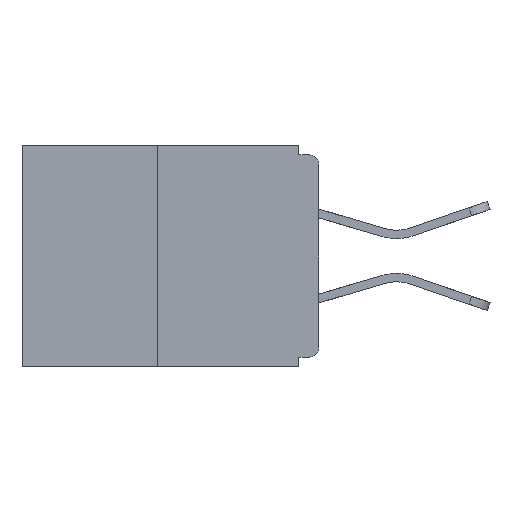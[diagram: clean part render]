
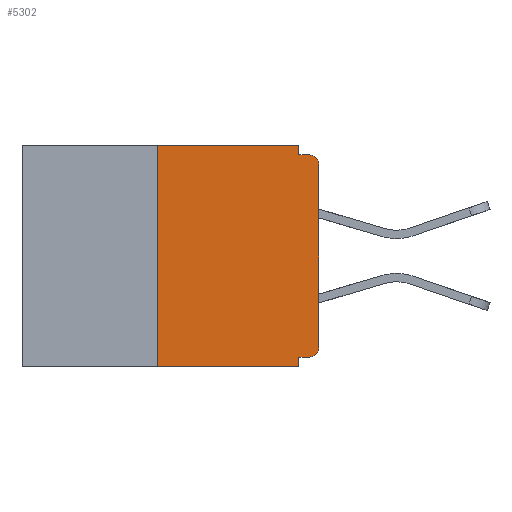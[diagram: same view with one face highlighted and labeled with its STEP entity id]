
A CAD part, left-side view. The second image highlights one B-rep face of the part: STEP entity #5302.
In plain terms, the highlighted planar face has unit normal (-1, 0, 0).
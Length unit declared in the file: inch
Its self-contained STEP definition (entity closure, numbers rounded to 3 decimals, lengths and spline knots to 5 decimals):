
#52 = EDGE_CURVE ( 'NONE', #6181, #1237, #245, .T. ) ;
#136 = DIRECTION ( 'NONE',  ( 0., 0., 1. ) ) ;
#245 = LINE ( 'NONE', #12150, #3765 ) ;
#295 = ORIENTED_EDGE ( 'NONE', *, *, #52, .T. ) ;
#482 = DIRECTION ( 'NONE',  ( 0., 0., -1. ) ) ;
#560 = EDGE_LOOP ( 'NONE', ( #10480, #6296, #295, #11154, #14332, #3397, #14997, #15441, #10477, #899 ) ) ;
#569 = VECTOR ( 'NONE', #6444, 39.37008 ) ;
#749 = VERTEX_POINT ( 'NONE', #13932 ) ;
#786 = CARTESIAN_POINT ( 'NONE',  ( 0., 0.015, -0.328 ) ) ;
#874 = EDGE_CURVE ( 'NONE', #11890, #1237, #2585, .T. ) ;
#875 = DIRECTION ( 'NONE',  ( 0., -1., 0. ) ) ;
#899 = ORIENTED_EDGE ( 'NONE', *, *, #11083, .F. ) ;
#1214 = VECTOR ( 'NONE', #12283, 39.37008 ) ;
#1237 = VERTEX_POINT ( 'NONE', #1892 ) ;
#1383 = EDGE_CURVE ( 'NONE', #6555, #16311, #5674, .T. ) ;
#1394 = PLANE ( 'NONE',  #5956 ) ;
#1415 = EDGE_CURVE ( 'NONE', #3898, #749, #15207, .T. ) ;
#1892 = CARTESIAN_POINT ( 'NONE',  ( 0., 0.031, -0.343 ) ) ;
#2345 = LINE ( 'NONE', #6497, #569 ) ;
#2422 = DIRECTION ( 'NONE',  ( 0., -1., 0. ) ) ;
#2491 = LINE ( 'NONE', #16131, #13175 ) ;
#2585 = LINE ( 'NONE', #4340, #9281 ) ;
#3397 = ORIENTED_EDGE ( 'NONE', *, *, #1415, .T. ) ;
#3548 = VERTEX_POINT ( 'NONE', #9812 ) ;
#3736 = EDGE_CURVE ( 'NONE', #5965, #3548, #2491, .T. ) ;
#3765 = VECTOR ( 'NONE', #875, 39.37008 ) ;
#3898 = VERTEX_POINT ( 'NONE', #786 ) ;
#3976 = CARTESIAN_POINT ( 'NONE',  ( 0., 0.031, 0. ) ) ;
#4182 = DIRECTION ( 'NONE',  ( 0., 0., -1. ) ) ;
#4340 = CARTESIAN_POINT ( 'NONE',  ( 0., 0.031, -0.343 ) ) ;
#5029 = CARTESIAN_POINT ( 'NONE',  ( 0., 0., -0.015 ) ) ;
#5181 = AXIS2_PLACEMENT_3D ( 'NONE', #15353, #12789, #10243 ) ;
#5302 = ADVANCED_FACE ( 'NONE', ( #13113 ), #1394, .F. ) ;
#5674 = LINE ( 'NONE', #5029, #13048 ) ;
#5956 = AXIS2_PLACEMENT_3D ( 'NONE', #7637, #6289, #11449 ) ;
#5965 = VERTEX_POINT ( 'NONE', #8681 ) ;
#6181 = VERTEX_POINT ( 'NONE', #10394 ) ;
#6289 = DIRECTION ( 'NONE',  ( 1., 0., 0. ) ) ;
#6296 = ORIENTED_EDGE ( 'NONE', *, *, #6857, .F. ) ;
#6430 = EDGE_CURVE ( 'NONE', #11897, #16311, #10716, .T. ) ;
#6444 = DIRECTION ( 'NONE',  ( 0., 1., 0. ) ) ;
#6497 = CARTESIAN_POINT ( 'NONE',  ( 0., 0., -0.328 ) ) ;
#6516 = CARTESIAN_POINT ( 'NONE',  ( 0., 0., 0. ) ) ;
#6555 = VERTEX_POINT ( 'NONE', #10830 ) ;
#6857 = EDGE_CURVE ( 'NONE', #6181, #5965, #15994, .T. ) ;
#7094 = CARTESIAN_POINT ( 'NONE',  ( 0., 0.015, -0.015 ) ) ;
#7215 = DIRECTION ( 'NONE',  ( 0., -1., 0. ) ) ;
#7637 = CARTESIAN_POINT ( 'NONE',  ( 0., 0.46, 0. ) ) ;
#8003 = DIRECTION ( 'NONE',  ( -1., 0., 0. ) ) ;
#8207 = EDGE_CURVE ( 'NONE', #3898, #11890, #2345, .T. ) ;
#8530 = VECTOR ( 'NONE', #11696, 39.37008 ) ;
#8681 = CARTESIAN_POINT ( 'NONE',  ( 0., 0.25, 0. ) ) ;
#8795 = CARTESIAN_POINT ( 'NONE',  ( 0., 0., -0.03 ) ) ;
#9281 = VECTOR ( 'NONE', #4182, 39.37008 ) ;
#9372 = AXIS2_PLACEMENT_3D ( 'NONE', #10521, #8003, #482 ) ;
#9812 = CARTESIAN_POINT ( 'NONE',  ( 0., 0.031, 0. ) ) ;
#9966 = CARTESIAN_POINT ( 'NONE',  ( 0., 0.25, 0. ) ) ;
#10243 = DIRECTION ( 'NONE',  ( 0., 0., -1. ) ) ;
#10394 = CARTESIAN_POINT ( 'NONE',  ( 0., 0.25, -0.343 ) ) ;
#10477 = ORIENTED_EDGE ( 'NONE', *, *, #1383, .F. ) ;
#10480 = ORIENTED_EDGE ( 'NONE', *, *, #3736, .F. ) ;
#10521 = CARTESIAN_POINT ( 'NONE',  ( 0., 0.015, -0.03 ) ) ;
#10716 = CIRCLE ( 'NONE', #9372, 0.015 ) ;
#10830 = CARTESIAN_POINT ( 'NONE',  ( 0., 0.031, -0.015 ) ) ;
#11083 = EDGE_CURVE ( 'NONE', #3548, #6555, #11346, .T. ) ;
#11154 = ORIENTED_EDGE ( 'NONE', *, *, #874, .F. ) ;
#11346 = LINE ( 'NONE', #3976, #8530 ) ;
#11449 = DIRECTION ( 'NONE',  ( 0., 0., -1. ) ) ;
#11696 = DIRECTION ( 'NONE',  ( 0., 0., -1. ) ) ;
#11843 = LINE ( 'NONE', #6516, #14185 ) ;
#11890 = VERTEX_POINT ( 'NONE', #12516 ) ;
#11897 = VERTEX_POINT ( 'NONE', #8795 ) ;
#12150 = CARTESIAN_POINT ( 'NONE',  ( 0., 0.46, -0.343 ) ) ;
#12283 = DIRECTION ( 'NONE',  ( 0., 0., 1. ) ) ;
#12516 = CARTESIAN_POINT ( 'NONE',  ( 0., 0.031, -0.328 ) ) ;
#12789 = DIRECTION ( 'NONE',  ( -1., 0., 0. ) ) ;
#13048 = VECTOR ( 'NONE', #2422, 39.37008 ) ;
#13113 = FACE_OUTER_BOUND ( 'NONE', #560, .T. ) ;
#13175 = VECTOR ( 'NONE', #7215, 39.37008 ) ;
#13932 = CARTESIAN_POINT ( 'NONE',  ( 0., 0., -0.313 ) ) ;
#14112 = EDGE_CURVE ( 'NONE', #749, #11897, #11843, .T. ) ;
#14185 = VECTOR ( 'NONE', #136, 39.37008 ) ;
#14332 = ORIENTED_EDGE ( 'NONE', *, *, #8207, .F. ) ;
#14997 = ORIENTED_EDGE ( 'NONE', *, *, #14112, .T. ) ;
#15207 = CIRCLE ( 'NONE', #5181, 0.015 ) ;
#15353 = CARTESIAN_POINT ( 'NONE',  ( 0., 0.015, -0.313 ) ) ;
#15441 = ORIENTED_EDGE ( 'NONE', *, *, #6430, .T. ) ;
#15994 = LINE ( 'NONE', #9966, #1214 ) ;
#16131 = CARTESIAN_POINT ( 'NONE',  ( 0., 0.46, 0. ) ) ;
#16311 = VERTEX_POINT ( 'NONE', #7094 ) ;
